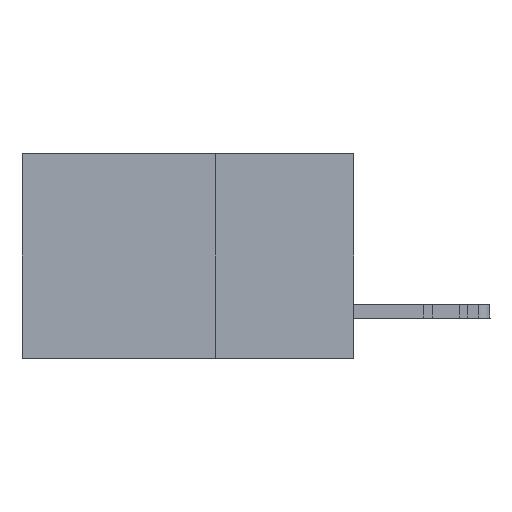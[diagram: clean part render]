
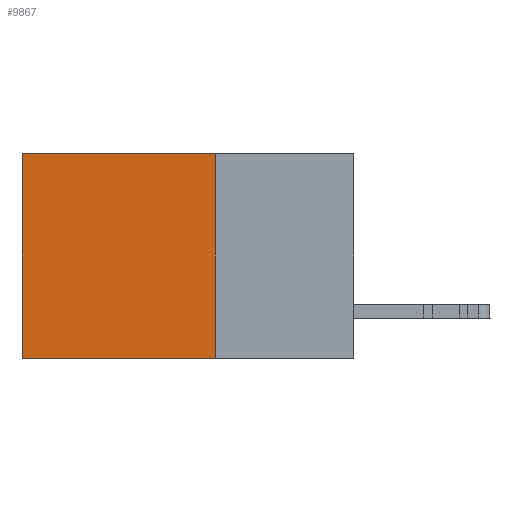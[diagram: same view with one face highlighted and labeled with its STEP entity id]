
A CAD part, left-side view. The second image highlights one B-rep face of the part: STEP entity #9867.
In plain terms, the highlighted planar face has unit normal (-1, 0, 0).
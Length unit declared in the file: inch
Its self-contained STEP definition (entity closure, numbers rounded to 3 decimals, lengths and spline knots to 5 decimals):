
#855 = DIRECTION ( 'NONE',  ( 1., 0., 0. ) ) ;
#1577 = VERTEX_POINT ( 'NONE', #32263 ) ;
#2216 = EDGE_CURVE ( 'NONE', #10593, #1577, #20389, .T. ) ;
#4154 = CARTESIAN_POINT ( 'NONE',  ( 0.2875, 0.25, 0. ) ) ;
#5133 = ORIENTED_EDGE ( 'NONE', *, *, #2216, .F. ) ;
#5164 = FACE_OUTER_BOUND ( 'NONE', #36084, .T. ) ;
#7037 = VECTOR ( 'NONE', #24462, 39.37008 ) ;
#8484 = VECTOR ( 'NONE', #35615, 39.37008 ) ;
#8636 = VERTEX_POINT ( 'NONE', #35744 ) ;
#9867 = ADVANCED_FACE ( 'NONE', ( #5164 ), #16947, .F. ) ;
#10593 = VERTEX_POINT ( 'NONE', #28825 ) ;
#11144 = EDGE_CURVE ( 'NONE', #1577, #8636, #15225, .T. ) ;
#11378 = CARTESIAN_POINT ( 'NONE',  ( 0.2875, 0.25, -0.37 ) ) ;
#13726 = VECTOR ( 'NONE', #14650, 39.37008 ) ;
#14650 = DIRECTION ( 'NONE',  ( 0., 1., 0. ) ) ;
#15225 = LINE ( 'NONE', #11378, #13726 ) ;
#16947 = PLANE ( 'NONE',  #33066 ) ;
#19805 = VERTEX_POINT ( 'NONE', #24284 ) ;
#20389 = LINE ( 'NONE', #4154, #39659 ) ;
#20755 = DIRECTION ( 'NONE',  ( 0., 0., -1. ) ) ;
#20810 = ORIENTED_EDGE ( 'NONE', *, *, #11144, .F. ) ;
#21225 = CARTESIAN_POINT ( 'NONE',  ( 0.2875, 0.25, 0. ) ) ;
#23714 = LINE ( 'NONE', #32079, #8484 ) ;
#24284 = CARTESIAN_POINT ( 'NONE',  ( 0.2875, 0.6, 0. ) ) ;
#24462 = DIRECTION ( 'NONE',  ( 0., 1., 0. ) ) ;
#28309 = LINE ( 'NONE', #21225, #7037 ) ;
#28825 = CARTESIAN_POINT ( 'NONE',  ( 0.2875, 0.25, 0. ) ) ;
#29500 = DIRECTION ( 'NONE',  ( 0., 0., -1. ) ) ;
#29862 = EDGE_CURVE ( 'NONE', #10593, #19805, #28309, .T. ) ;
#29921 = CARTESIAN_POINT ( 'NONE',  ( 0.2875, 0.25, 0. ) ) ;
#30682 = EDGE_CURVE ( 'NONE', #19805, #8636, #23714, .T. ) ;
#31157 = ORIENTED_EDGE ( 'NONE', *, *, #29862, .T. ) ;
#32079 = CARTESIAN_POINT ( 'NONE',  ( 0.2875, 0.6, 0. ) ) ;
#32263 = CARTESIAN_POINT ( 'NONE',  ( 0.2875, 0.25, -0.37 ) ) ;
#33066 = AXIS2_PLACEMENT_3D ( 'NONE', #29921, #855, #29500 ) ;
#35615 = DIRECTION ( 'NONE',  ( 0., 0., -1. ) ) ;
#35744 = CARTESIAN_POINT ( 'NONE',  ( 0.2875, 0.6, -0.37 ) ) ;
#36084 = EDGE_LOOP ( 'NONE', ( #40585, #20810, #5133, #31157 ) ) ;
#39659 = VECTOR ( 'NONE', #20755, 39.37008 ) ;
#40585 = ORIENTED_EDGE ( 'NONE', *, *, #30682, .T. ) ;
